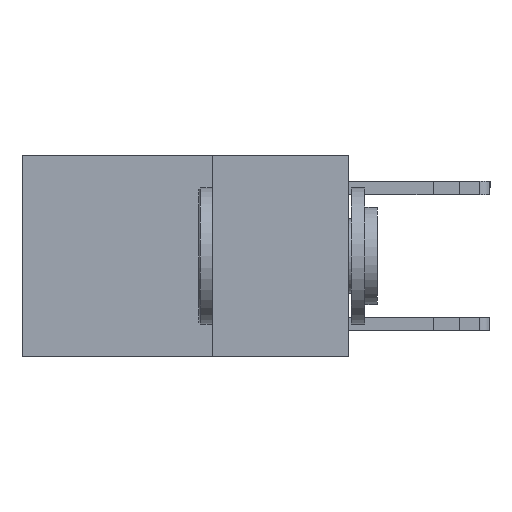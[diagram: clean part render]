
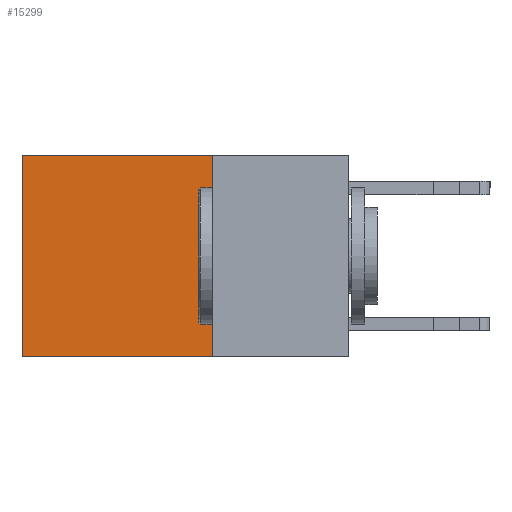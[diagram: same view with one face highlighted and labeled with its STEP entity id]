
A CAD part, left-side view. The second image highlights one B-rep face of the part: STEP entity #15299.
In plain terms, the highlighted planar face has unit normal (-1, 0, 0).
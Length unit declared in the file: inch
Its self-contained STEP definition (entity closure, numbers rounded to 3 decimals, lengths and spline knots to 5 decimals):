
#195 = LINE ( 'NONE', #6837, #15038 ) ;
#549 = VERTEX_POINT ( 'NONE', #1445 ) ;
#832 = DIRECTION ( 'NONE',  ( 0., 1., 0. ) ) ;
#911 = EDGE_CURVE ( 'NONE', #5097, #549, #6485, .T. ) ;
#1111 = VECTOR ( 'NONE', #832, 39.37008 ) ;
#1445 = CARTESIAN_POINT ( 'NONE',  ( 0.2625, 0.6, 0. ) ) ;
#2465 = DIRECTION ( 'NONE',  ( 0., 0., -1. ) ) ;
#2510 = CARTESIAN_POINT ( 'NONE',  ( 0.2625, 0.25, -0.37 ) ) ;
#2562 = VERTEX_POINT ( 'NONE', #2510 ) ;
#2786 = PLANE ( 'NONE',  #5324 ) ;
#5097 = VERTEX_POINT ( 'NONE', #8993 ) ;
#5324 = AXIS2_PLACEMENT_3D ( 'NONE', #8207, #7037, #13687 ) ;
#5438 = VERTEX_POINT ( 'NONE', #10415 ) ;
#5552 = EDGE_CURVE ( 'NONE', #2562, #5438, #8428, .T. ) ;
#6485 = LINE ( 'NONE', #8767, #1111 ) ;
#6694 = VECTOR ( 'NONE', #13910, 39.37008 ) ;
#6837 = CARTESIAN_POINT ( 'NONE',  ( 0.2625, 0.25, 0. ) ) ;
#6841 = EDGE_CURVE ( 'NONE', #549, #5438, #14099, .T. ) ;
#7037 = DIRECTION ( 'NONE',  ( 1., 0., 0. ) ) ;
#7094 = CARTESIAN_POINT ( 'NONE',  ( 0.2625, 0.25, -0.37 ) ) ;
#8207 = CARTESIAN_POINT ( 'NONE',  ( 0.2625, 0.25, 0. ) ) ;
#8242 = DIRECTION ( 'NONE',  ( 0., 0., -1. ) ) ;
#8428 = LINE ( 'NONE', #7094, #6694 ) ;
#8626 = ORIENTED_EDGE ( 'NONE', *, *, #6841, .T. ) ;
#8767 = CARTESIAN_POINT ( 'NONE',  ( 0.2625, 0.25, 0. ) ) ;
#8993 = CARTESIAN_POINT ( 'NONE',  ( 0.2625, 0.25, 0. ) ) ;
#9864 = ORIENTED_EDGE ( 'NONE', *, *, #5552, .F. ) ;
#10415 = CARTESIAN_POINT ( 'NONE',  ( 0.2625, 0.6, -0.37 ) ) ;
#10465 = ORIENTED_EDGE ( 'NONE', *, *, #14321, .F. ) ;
#10640 = VECTOR ( 'NONE', #2465, 39.37008 ) ;
#10980 = FACE_OUTER_BOUND ( 'NONE', #11777, .T. ) ;
#11777 = EDGE_LOOP ( 'NONE', ( #8626, #9864, #10465, #14574 ) ) ;
#13687 = DIRECTION ( 'NONE',  ( 0., 0., -1. ) ) ;
#13910 = DIRECTION ( 'NONE',  ( 0., 1., 0. ) ) ;
#14099 = LINE ( 'NONE', #14696, #10640 ) ;
#14321 = EDGE_CURVE ( 'NONE', #5097, #2562, #195, .T. ) ;
#14574 = ORIENTED_EDGE ( 'NONE', *, *, #911, .T. ) ;
#14696 = CARTESIAN_POINT ( 'NONE',  ( 0.2625, 0.6, 0. ) ) ;
#15038 = VECTOR ( 'NONE', #8242, 39.37008 ) ;
#15299 = ADVANCED_FACE ( 'NONE', ( #10980 ), #2786, .F. ) ;
